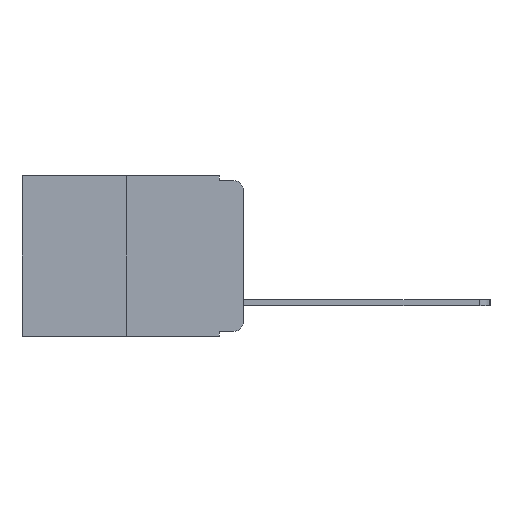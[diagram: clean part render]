
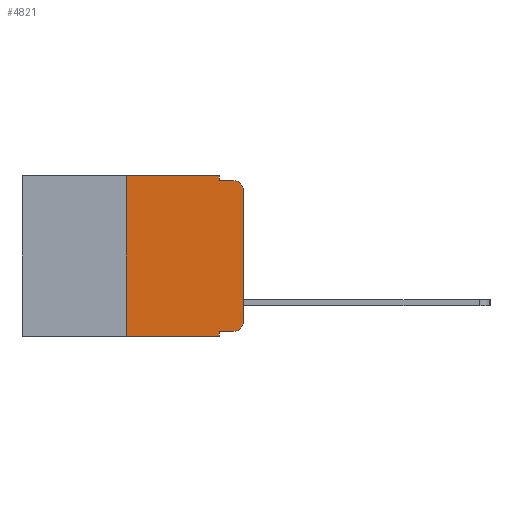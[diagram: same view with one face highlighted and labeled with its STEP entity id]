
A CAD part, left-side view. The second image highlights one B-rep face of the part: STEP entity #4821.
In plain terms, the highlighted planar face has unit normal (-1, 0, 0).
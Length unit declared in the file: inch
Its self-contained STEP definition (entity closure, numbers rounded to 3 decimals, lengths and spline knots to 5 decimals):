
#321 = VECTOR ( 'NONE', #18360, 39.37008 ) ;
#329 = CARTESIAN_POINT ( 'NONE',  ( 0., 0.02, -0.313 ) ) ;
#799 = CARTESIAN_POINT ( 'NONE',  ( 0., 0.051, -0.01 ) ) ;
#952 = EDGE_CURVE ( 'NONE', #22942, #6820, #17851, .T. ) ;
#1046 = FACE_OUTER_BOUND ( 'NONE', #3899, .T. ) ;
#1394 = ORIENTED_EDGE ( 'NONE', *, *, #14425, .F. ) ;
#1523 = VECTOR ( 'NONE', #12394, 39.37008 ) ;
#1556 = CARTESIAN_POINT ( 'NONE',  ( 0., 0.051, -0.01 ) ) ;
#1841 = AXIS2_PLACEMENT_3D ( 'NONE', #23639, #3095, #16352 ) ;
#2443 = CARTESIAN_POINT ( 'NONE',  ( 0., 0.051, -0.333 ) ) ;
#2696 = CARTESIAN_POINT ( 'NONE',  ( 0., 0.051, -0.343 ) ) ;
#2809 = DIRECTION ( 'NONE',  ( 0., -1., 0. ) ) ;
#3095 = DIRECTION ( 'NONE',  ( 1., 0., 0. ) ) ;
#3243 = ORIENTED_EDGE ( 'NONE', *, *, #11890, .F. ) ;
#3481 = CARTESIAN_POINT ( 'NONE',  ( 0., 0.02, -0.03 ) ) ;
#3822 = DIRECTION ( 'NONE',  ( 0., -1., 0. ) ) ;
#3899 = EDGE_LOOP ( 'NONE', ( #10425, #15429, #1394, #7158, #12203, #3243, #8338, #8950, #13984, #14568 ) ) ;
#4173 = CIRCLE ( 'NONE', #5596, 0.02 ) ;
#4821 = ADVANCED_FACE ( 'NONE', ( #1046 ), #21799, .F. ) ;
#4968 = LINE ( 'NONE', #17967, #19339 ) ;
#5445 = DIRECTION ( 'NONE',  ( 0., 0., -1. ) ) ;
#5596 = AXIS2_PLACEMENT_3D ( 'NONE', #3481, #16725, #5445 ) ;
#5652 = VECTOR ( 'NONE', #14014, 39.37008 ) ;
#5744 = LINE ( 'NONE', #799, #20116 ) ;
#6072 = LINE ( 'NONE', #23411, #1523 ) ;
#6410 = CIRCLE ( 'NONE', #18060, 0.02 ) ;
#6680 = VERTEX_POINT ( 'NONE', #19307 ) ;
#6790 = EDGE_CURVE ( 'NONE', #6680, #16813, #6410, .T. ) ;
#6820 = VERTEX_POINT ( 'NONE', #23686 ) ;
#6821 = VERTEX_POINT ( 'NONE', #11591 ) ;
#7158 = ORIENTED_EDGE ( 'NONE', *, *, #13186, .F. ) ;
#7208 = LINE ( 'NONE', #8090, #16624 ) ;
#7821 = CARTESIAN_POINT ( 'NONE',  ( 0., 0.473, 0. ) ) ;
#8073 = EDGE_CURVE ( 'NONE', #15993, #6680, #15702, .T. ) ;
#8090 = CARTESIAN_POINT ( 'NONE',  ( 0., 0.051, 0. ) ) ;
#8338 = ORIENTED_EDGE ( 'NONE', *, *, #21363, .T. ) ;
#8390 = DIRECTION ( 'NONE',  ( 0., -1., 0. ) ) ;
#8942 = VERTEX_POINT ( 'NONE', #16555 ) ;
#8950 = ORIENTED_EDGE ( 'NONE', *, *, #10637, .F. ) ;
#8953 = VECTOR ( 'NONE', #3822, 39.37008 ) ;
#9509 = CARTESIAN_POINT ( 'NONE',  ( 0., 0.473, -0.343 ) ) ;
#10425 = ORIENTED_EDGE ( 'NONE', *, *, #16907, .T. ) ;
#10627 = LINE ( 'NONE', #16504, #321 ) ;
#10637 = EDGE_CURVE ( 'NONE', #15993, #19479, #4968, .T. ) ;
#11591 = CARTESIAN_POINT ( 'NONE',  ( 0., 0., -0.03 ) ) ;
#11864 = CARTESIAN_POINT ( 'NONE',  ( 0., 0.25, 0. ) ) ;
#11890 = EDGE_CURVE ( 'NONE', #8942, #22942, #6072, .T. ) ;
#12203 = ORIENTED_EDGE ( 'NONE', *, *, #952, .F. ) ;
#12394 = DIRECTION ( 'NONE',  ( 0., 0., 1. ) ) ;
#12946 = VECTOR ( 'NONE', #8390, 39.37008 ) ;
#13186 = EDGE_CURVE ( 'NONE', #6820, #17976, #7208, .T. ) ;
#13639 = CARTESIAN_POINT ( 'NONE',  ( 0., 0.02, -0.01 ) ) ;
#13984 = ORIENTED_EDGE ( 'NONE', *, *, #8073, .T. ) ;
#14014 = DIRECTION ( 'NONE',  ( 0., -1., 0. ) ) ;
#14425 = EDGE_CURVE ( 'NONE', #17976, #22879, #5744, .T. ) ;
#14568 = ORIENTED_EDGE ( 'NONE', *, *, #6790, .T. ) ;
#15429 = ORIENTED_EDGE ( 'NONE', *, *, #15670, .T. ) ;
#15670 = EDGE_CURVE ( 'NONE', #6821, #22879, #4173, .T. ) ;
#15702 = LINE ( 'NONE', #17728, #5652 ) ;
#15993 = VERTEX_POINT ( 'NONE', #2443 ) ;
#16270 = CARTESIAN_POINT ( 'NONE',  ( 0., 0., -0.313 ) ) ;
#16352 = DIRECTION ( 'NONE',  ( 0., 0., -1. ) ) ;
#16504 = CARTESIAN_POINT ( 'NONE',  ( 0., 0., 0. ) ) ;
#16555 = CARTESIAN_POINT ( 'NONE',  ( 0., 0.25, -0.343 ) ) ;
#16624 = VECTOR ( 'NONE', #22951, 39.37008 ) ;
#16725 = DIRECTION ( 'NONE',  ( -1., 0., 0. ) ) ;
#16813 = VERTEX_POINT ( 'NONE', #16270 ) ;
#16907 = EDGE_CURVE ( 'NONE', #16813, #6821, #10627, .T. ) ;
#17067 = DIRECTION ( 'NONE',  ( 0., 0., -1. ) ) ;
#17728 = CARTESIAN_POINT ( 'NONE',  ( 0., 0.051, -0.333 ) ) ;
#17851 = LINE ( 'NONE', #7821, #12946 ) ;
#17967 = CARTESIAN_POINT ( 'NONE',  ( 0., 0.051, 0. ) ) ;
#17976 = VERTEX_POINT ( 'NONE', #1556 ) ;
#18060 = AXIS2_PLACEMENT_3D ( 'NONE', #329, #19787, #17067 ) ;
#18360 = DIRECTION ( 'NONE',  ( 0., 0., 1. ) ) ;
#19307 = CARTESIAN_POINT ( 'NONE',  ( 0., 0.02, -0.333 ) ) ;
#19339 = VECTOR ( 'NONE', #19815, 39.37008 ) ;
#19479 = VERTEX_POINT ( 'NONE', #2696 ) ;
#19787 = DIRECTION ( 'NONE',  ( -1., 0., 0. ) ) ;
#19815 = DIRECTION ( 'NONE',  ( 0., 0., -1. ) ) ;
#20116 = VECTOR ( 'NONE', #2809, 39.37008 ) ;
#21363 = EDGE_CURVE ( 'NONE', #8942, #19479, #23756, .T. ) ;
#21799 = PLANE ( 'NONE',  #1841 ) ;
#22879 = VERTEX_POINT ( 'NONE', #13639 ) ;
#22942 = VERTEX_POINT ( 'NONE', #11864 ) ;
#22951 = DIRECTION ( 'NONE',  ( 0., 0., -1. ) ) ;
#23411 = CARTESIAN_POINT ( 'NONE',  ( 0., 0.25, 0. ) ) ;
#23639 = CARTESIAN_POINT ( 'NONE',  ( 0., 0.473, 0. ) ) ;
#23686 = CARTESIAN_POINT ( 'NONE',  ( 0., 0.051, 0. ) ) ;
#23756 = LINE ( 'NONE', #9509, #8953 ) ;
